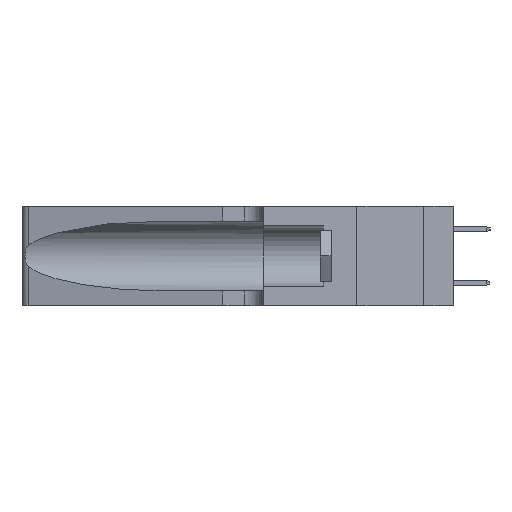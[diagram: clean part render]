
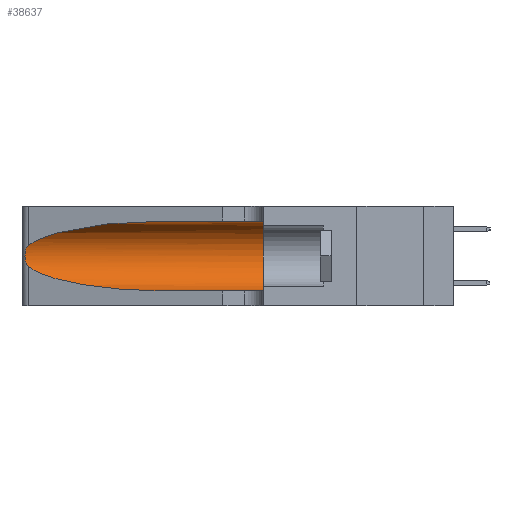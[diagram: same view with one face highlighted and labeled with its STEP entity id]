
A CAD part, left-side view. The second image highlights one B-rep face of the part: STEP entity #38637.
In plain terms, the highlighted cylindrical face has radius 3.308 mm (diameter 6.617 mm), a partial arc.
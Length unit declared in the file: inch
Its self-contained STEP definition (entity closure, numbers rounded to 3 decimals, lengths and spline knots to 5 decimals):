
#192 = CARTESIAN_POINT ( 'NONE',  ( 0.25487, 1.22718, 0.22369 ) ) ;
#719 = CARTESIAN_POINT ( 'NONE',  ( 0.25555, 1.22994, 0.2215 ) ) ;
#847 = VERTEX_POINT ( 'NONE', #34114 ) ;
#982 =( BOUNDED_CURVE ( )  B_SPLINE_CURVE ( 3, ( #17243, #14090, #21344, #31972 ),
 .UNSPECIFIED., .F., .F. ) 
 B_SPLINE_CURVE_WITH_KNOTS ( ( 4, 4 ),
 ( 3.44316, 4.71239 ),
 .UNSPECIFIED. ) 
 CURVE ( )  GEOMETRIC_REPRESENTATION_ITEM ( )  RATIONAL_B_SPLINE_CURVE ( ( 1., 0.87, 0.87, 1. ) ) 
 REPRESENTATION_ITEM ( '' )  );
#2200 = EDGE_CURVE ( 'NONE', #30191, #18455, #35540, .T. ) ;
#2560 = CARTESIAN_POINT ( 'NONE',  ( 0.25789, 1.23486, 0.15765 ) ) ;
#2776 = CYLINDRICAL_SURFACE ( 'NONE', #8848, 0.13025 ) ;
#3267 = CARTESIAN_POINT ( 'NONE',  ( 0.25856, 1.23593, 0.16098 ) ) ;
#4093 = CARTESIAN_POINT ( 'NONE',  ( 0.25487, 1.22718, 0.14631 ) ) ;
#4442 = CARTESIAN_POINT ( 'NONE',  ( 0.1305, 0.72297, 0.31525 ) ) ;
#5739 = AXIS2_PLACEMENT_3D ( 'NONE', #40394, #28564, #11180 ) ;
#6976 = CARTESIAN_POINT ( 'NONE',  ( 0.2373, 1.15595, 0.28018 ) ) ;
#8567 = CARTESIAN_POINT ( 'NONE',  ( 0.25487, 1.22718, 0.22369 ) ) ;
#8848 = AXIS2_PLACEMENT_3D ( 'NONE', #20657, #38776, #27660 ) ;
#9110 = CARTESIAN_POINT ( 'NONE',  ( 0.25854, 1.2359, 0.20912 ) ) ;
#11180 = DIRECTION ( 'NONE',  ( 0., 0., 1. ) ) ;
#13208 = CARTESIAN_POINT ( 'NONE',  ( 0.26018, 1.23835, 0.19895 ) ) ;
#13353 = ORIENTED_EDGE ( 'NONE', *, *, #2200, .T. ) ;
#13909 = CARTESIAN_POINT ( 'NONE',  ( 0.25487, 1.22718, 0.14631 ) ) ;
#14090 = CARTESIAN_POINT ( 'NONE',  ( 0.2373, 1.15595, 0.08982 ) ) ;
#15763 = CIRCLE ( 'NONE', #5739, 0.13025 ) ;
#17243 = CARTESIAN_POINT ( 'NONE',  ( 0.25487, 1.22718, 0.14631 ) ) ;
#18405 = ORIENTED_EDGE ( 'NONE', *, *, #26760, .T. ) ;
#18455 = VERTEX_POINT ( 'NONE', #25050 ) ;
#18890 = B_SPLINE_CURVE_WITH_KNOTS ( 'NONE', 3,
 ( #34056, #719, #42189, #38803, #9110, #13208, #27922, #46522, #26320, #3267, #2560, #36601, #35884, #13909 ),
 .UNSPECIFIED., .F., .F.,
 ( 4, 2, 2, 2, 2, 2, 4 ),
 ( 0., 0.00027, 0.00053, 0.00107, 0.0016, 0.00187, 0.00214 ),
 .UNSPECIFIED. ) ;
#20657 = CARTESIAN_POINT ( 'NONE',  ( 0.1305, 1.61858, 0.185 ) ) ;
#21029 = ORIENTED_EDGE ( 'NONE', *, *, #27254, .F. ) ;
#21344 = CARTESIAN_POINT ( 'NONE',  ( 0.18966, 0.96281, 0.05475 ) ) ;
#22934 = VERTEX_POINT ( 'NONE', #4442 ) ;
#25050 = CARTESIAN_POINT ( 'NONE',  ( 0.1305, 0.35, 0.05475 ) ) ;
#26320 = CARTESIAN_POINT ( 'NONE',  ( 0.26017, 1.23833, 0.17102 ) ) ;
#26760 = EDGE_CURVE ( 'NONE', #45001, #30191, #982, .T. ) ;
#27254 = EDGE_CURVE ( 'NONE', #847, #18455, #15763, .T. ) ;
#27650 = CARTESIAN_POINT ( 'NONE',  ( 0.1305, 0.72297, 0.05475 ) ) ;
#27660 = DIRECTION ( 'NONE',  ( 0., 0., -1. ) ) ;
#27922 = CARTESIAN_POINT ( 'NONE',  ( 0.26075, 1.23896, 0.19203 ) ) ;
#28564 = DIRECTION ( 'NONE',  ( 0., 1., 0. ) ) ;
#29925 = EDGE_CURVE ( 'NONE', #22934, #847, #40004, .T. ) ;
#30191 = VERTEX_POINT ( 'NONE', #27650 ) ;
#31972 = CARTESIAN_POINT ( 'NONE',  ( 0.1305, 0.72297, 0.05475 ) ) ;
#32223 = FACE_OUTER_BOUND ( 'NONE', #39436, .T. ) ;
#32293 = EDGE_CURVE ( 'NONE', #22934, #41944, #40192, .T. ) ;
#33725 = ORIENTED_EDGE ( 'NONE', *, *, #32293, .T. ) ;
#33955 = ORIENTED_EDGE ( 'NONE', *, *, #29925, .F. ) ;
#34056 = CARTESIAN_POINT ( 'NONE',  ( 0.25487, 1.22718, 0.22369 ) ) ;
#34114 = CARTESIAN_POINT ( 'NONE',  ( 0.1305, 0.35, 0.31525 ) ) ;
#35540 = LINE ( 'NONE', #42553, #36552 ) ;
#35884 = CARTESIAN_POINT ( 'NONE',  ( 0.25555, 1.22993, 0.14849 ) ) ;
#36552 = VECTOR ( 'NONE', #36730, 39.37008 ) ;
#36601 = CARTESIAN_POINT ( 'NONE',  ( 0.25639, 1.23186, 0.15144 ) ) ;
#36730 = DIRECTION ( 'NONE',  ( 0., -1., 0. ) ) ;
#37152 = CARTESIAN_POINT ( 'NONE',  ( 0.18966, 0.96281, 0.31525 ) ) ;
#38637 = ADVANCED_FACE ( 'NONE', ( #32223 ), #2776, .F. ) ;
#38776 = DIRECTION ( 'NONE',  ( 0., -1., 0. ) ) ;
#38803 = CARTESIAN_POINT ( 'NONE',  ( 0.25787, 1.23484, 0.2124 ) ) ;
#38963 = ORIENTED_EDGE ( 'NONE', *, *, #47033, .T. ) ;
#39092 = VECTOR ( 'NONE', #39532, 39.37008 ) ;
#39436 = EDGE_LOOP ( 'NONE', ( #33725, #38963, #18405, #13353, #21029, #33955 ) ) ;
#39532 = DIRECTION ( 'NONE',  ( 0., -1., 0. ) ) ;
#39813 = CARTESIAN_POINT ( 'NONE',  ( 0.1305, 0.72297, 0.31525 ) ) ;
#40004 = LINE ( 'NONE', #44112, #39092 ) ;
#40192 =( BOUNDED_CURVE ( )  B_SPLINE_CURVE ( 3, ( #39813, #37152, #6976, #192 ),
 .UNSPECIFIED., .F., .F. ) 
 B_SPLINE_CURVE_WITH_KNOTS ( ( 4, 4 ),
 ( 1.5708, 2.84003 ),
 .UNSPECIFIED. ) 
 CURVE ( )  GEOMETRIC_REPRESENTATION_ITEM ( )  RATIONAL_B_SPLINE_CURVE ( ( 1., 0.87, 0.87, 1. ) ) 
 REPRESENTATION_ITEM ( '' )  );
#40394 = CARTESIAN_POINT ( 'NONE',  ( 0.1305, 0.35, 0.185 ) ) ;
#41944 = VERTEX_POINT ( 'NONE', #8567 ) ;
#42189 = CARTESIAN_POINT ( 'NONE',  ( 0.25639, 1.23184, 0.21858 ) ) ;
#42553 = CARTESIAN_POINT ( 'NONE',  ( 0.1305, 1.61858, 0.05475 ) ) ;
#44112 = CARTESIAN_POINT ( 'NONE',  ( 0.1305, 1.61858, 0.31525 ) ) ;
#45001 = VERTEX_POINT ( 'NONE', #4093 ) ;
#46522 = CARTESIAN_POINT ( 'NONE',  ( 0.26075, 1.23896, 0.178 ) ) ;
#47033 = EDGE_CURVE ( 'NONE', #41944, #45001, #18890, .T. ) ;
